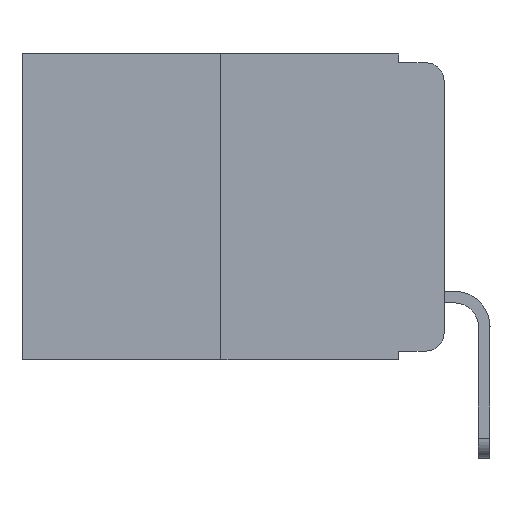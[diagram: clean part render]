
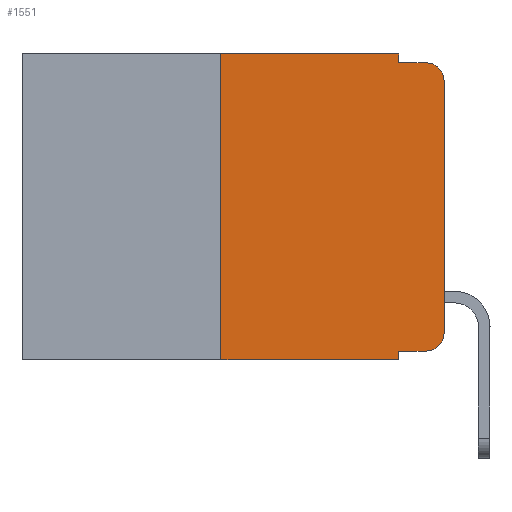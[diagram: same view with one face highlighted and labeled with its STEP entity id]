
A CAD part, left-side view. The second image highlights one B-rep face of the part: STEP entity #1551.
In plain terms, the highlighted planar face has unit normal (-1, 0, 0).
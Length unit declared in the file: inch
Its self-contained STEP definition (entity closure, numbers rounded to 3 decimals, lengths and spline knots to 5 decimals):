
#377 = CARTESIAN_POINT ( 'NONE',  ( 0., 0.051, -0.01 ) ) ;
#551 = CARTESIAN_POINT ( 'NONE',  ( 0., 0.02, -0.333 ) ) ;
#581 = CARTESIAN_POINT ( 'NONE',  ( 0., 0.473, -0.343 ) ) ;
#866 = EDGE_CURVE ( 'NONE', #14477, #10814, #18316, .T. ) ;
#1181 = LINE ( 'NONE', #4937, #20883 ) ;
#1551 = ADVANCED_FACE ( 'NONE', ( #23751 ), #15836, .F. ) ;
#1585 = EDGE_CURVE ( 'NONE', #14540, #8700, #23374, .T. ) ;
#1736 = ORIENTED_EDGE ( 'NONE', *, *, #2843, .T. ) ;
#2041 = DIRECTION ( 'NONE',  ( -1., 0., 0. ) ) ;
#2245 = AXIS2_PLACEMENT_3D ( 'NONE', #3662, #23142, #21274 ) ;
#2323 = CARTESIAN_POINT ( 'NONE',  ( 0., 0., -0.03 ) ) ;
#2755 = CARTESIAN_POINT ( 'NONE',  ( 0., 0.473, 0. ) ) ;
#2843 = EDGE_CURVE ( 'NONE', #19905, #6173, #13609, .T. ) ;
#3216 = DIRECTION ( 'NONE',  ( 0., -1., 0. ) ) ;
#3662 = CARTESIAN_POINT ( 'NONE',  ( 0., 0.02, -0.03 ) ) ;
#4937 = CARTESIAN_POINT ( 'NONE',  ( 0., 0.051, 0. ) ) ;
#5417 = VECTOR ( 'NONE', #17762, 39.37008 ) ;
#6173 = VERTEX_POINT ( 'NONE', #2323 ) ;
#6267 = DIRECTION ( 'NONE',  ( 0., 0., -1. ) ) ;
#6585 = LINE ( 'NONE', #14276, #14856 ) ;
#6665 = EDGE_CURVE ( 'NONE', #10814, #14540, #13849, .T. ) ;
#7012 = ORIENTED_EDGE ( 'NONE', *, *, #6665, .F. ) ;
#8074 = ORIENTED_EDGE ( 'NONE', *, *, #14268, .T. ) ;
#8083 = DIRECTION ( 'NONE',  ( 0., 0., 1. ) ) ;
#8700 = VERTEX_POINT ( 'NONE', #18146 ) ;
#8996 = EDGE_CURVE ( 'NONE', #6173, #8700, #16701, .T. ) ;
#9095 = ORIENTED_EDGE ( 'NONE', *, *, #8996, .T. ) ;
#9832 = CARTESIAN_POINT ( 'NONE',  ( 0., 0., 0. ) ) ;
#10070 = CARTESIAN_POINT ( 'NONE',  ( 0., 0.051, 0. ) ) ;
#10124 = LINE ( 'NONE', #581, #19087 ) ;
#10340 = VECTOR ( 'NONE', #3216, 39.37008 ) ;
#10395 = CIRCLE ( 'NONE', #22842, 0.02 ) ;
#10526 = ORIENTED_EDGE ( 'NONE', *, *, #23957, .T. ) ;
#10549 = ORIENTED_EDGE ( 'NONE', *, *, #20734, .F. ) ;
#10814 = VERTEX_POINT ( 'NONE', #16323 ) ;
#11377 = VECTOR ( 'NONE', #19225, 39.37008 ) ;
#11765 = DIRECTION ( 'NONE',  ( 0., -1., 0. ) ) ;
#12516 = AXIS2_PLACEMENT_3D ( 'NONE', #2755, #23504, #6267 ) ;
#12697 = VECTOR ( 'NONE', #8083, 39.37008 ) ;
#12992 = CARTESIAN_POINT ( 'NONE',  ( 0., 0.051, -0.333 ) ) ;
#13244 = CARTESIAN_POINT ( 'NONE',  ( 0., 0.02, -0.313 ) ) ;
#13434 = CARTESIAN_POINT ( 'NONE',  ( 0., 0.25, 0. ) ) ;
#13609 = LINE ( 'NONE', #9832, #12697 ) ;
#13849 = LINE ( 'NONE', #10070, #5417 ) ;
#13951 = DIRECTION ( 'NONE',  ( 0., -1., 0. ) ) ;
#14171 = CARTESIAN_POINT ( 'NONE',  ( 0., 0., -0.313 ) ) ;
#14268 = EDGE_CURVE ( 'NONE', #17205, #24603, #6585, .T. ) ;
#14276 = CARTESIAN_POINT ( 'NONE',  ( 0., 0.051, -0.333 ) ) ;
#14443 = EDGE_LOOP ( 'NONE', ( #1736, #9095, #19684, #7012, #23749, #10549, #10526, #19037, #8074, #15328 ) ) ;
#14477 = VERTEX_POINT ( 'NONE', #16930 ) ;
#14540 = VERTEX_POINT ( 'NONE', #15757 ) ;
#14789 = CARTESIAN_POINT ( 'NONE',  ( 0., 0.473, 0. ) ) ;
#14856 = VECTOR ( 'NONE', #18423, 39.37008 ) ;
#15201 = LINE ( 'NONE', #13434, #11377 ) ;
#15328 = ORIENTED_EDGE ( 'NONE', *, *, #16167, .T. ) ;
#15757 = CARTESIAN_POINT ( 'NONE',  ( 0., 0.051, -0.01 ) ) ;
#15836 = PLANE ( 'NONE',  #12516 ) ;
#16032 = CARTESIAN_POINT ( 'NONE',  ( 0., 0.25, -0.343 ) ) ;
#16167 = EDGE_CURVE ( 'NONE', #24603, #19905, #10395, .T. ) ;
#16323 = CARTESIAN_POINT ( 'NONE',  ( 0., 0.051, 0. ) ) ;
#16701 = CIRCLE ( 'NONE', #2245, 0.02 ) ;
#16930 = CARTESIAN_POINT ( 'NONE',  ( 0., 0.25, 0. ) ) ;
#17205 = VERTEX_POINT ( 'NONE', #12992 ) ;
#17224 = EDGE_CURVE ( 'NONE', #17205, #20215, #1181, .T. ) ;
#17762 = DIRECTION ( 'NONE',  ( 0., 0., -1. ) ) ;
#18146 = CARTESIAN_POINT ( 'NONE',  ( 0., 0.02, -0.01 ) ) ;
#18316 = LINE ( 'NONE', #14789, #10340 ) ;
#18423 = DIRECTION ( 'NONE',  ( 0., -1., 0. ) ) ;
#19037 = ORIENTED_EDGE ( 'NONE', *, *, #17224, .F. ) ;
#19087 = VECTOR ( 'NONE', #11765, 39.37008 ) ;
#19225 = DIRECTION ( 'NONE',  ( 0., 0., 1. ) ) ;
#19684 = ORIENTED_EDGE ( 'NONE', *, *, #1585, .F. ) ;
#19905 = VERTEX_POINT ( 'NONE', #14171 ) ;
#20215 = VERTEX_POINT ( 'NONE', #20541 ) ;
#20541 = CARTESIAN_POINT ( 'NONE',  ( 0., 0.051, -0.343 ) ) ;
#20734 = EDGE_CURVE ( 'NONE', #23939, #14477, #15201, .T. ) ;
#20883 = VECTOR ( 'NONE', #22545, 39.37008 ) ;
#21274 = DIRECTION ( 'NONE',  ( 0., 0., -1. ) ) ;
#22541 = DIRECTION ( 'NONE',  ( 0., 0., -1. ) ) ;
#22545 = DIRECTION ( 'NONE',  ( 0., 0., -1. ) ) ;
#22842 = AXIS2_PLACEMENT_3D ( 'NONE', #13244, #2041, #22541 ) ;
#23142 = DIRECTION ( 'NONE',  ( -1., 0., 0. ) ) ;
#23374 = LINE ( 'NONE', #377, #23777 ) ;
#23504 = DIRECTION ( 'NONE',  ( 1., 0., 0. ) ) ;
#23749 = ORIENTED_EDGE ( 'NONE', *, *, #866, .F. ) ;
#23751 = FACE_OUTER_BOUND ( 'NONE', #14443, .T. ) ;
#23777 = VECTOR ( 'NONE', #13951, 39.37008 ) ;
#23939 = VERTEX_POINT ( 'NONE', #16032 ) ;
#23957 = EDGE_CURVE ( 'NONE', #23939, #20215, #10124, .T. ) ;
#24603 = VERTEX_POINT ( 'NONE', #551 ) ;
